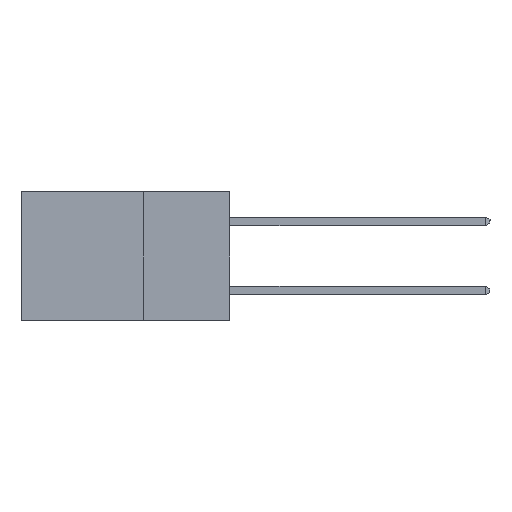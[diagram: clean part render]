
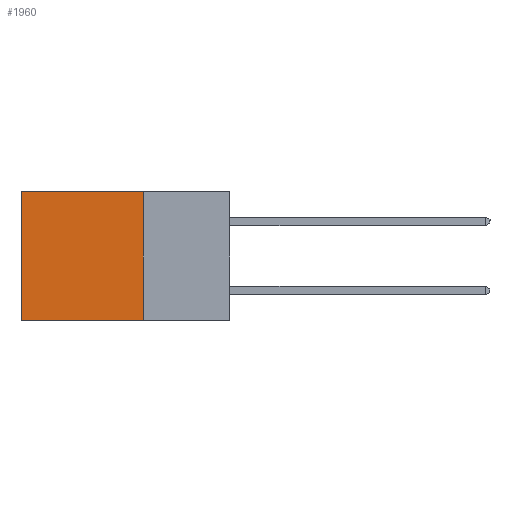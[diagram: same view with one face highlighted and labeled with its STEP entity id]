
A CAD part, left-side view. The second image highlights one B-rep face of the part: STEP entity #1960.
In plain terms, the highlighted planar face has unit normal (-1, 0, 0).
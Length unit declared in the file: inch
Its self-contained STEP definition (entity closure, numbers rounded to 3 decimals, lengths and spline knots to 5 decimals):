
#203 = EDGE_CURVE ( 'NONE', #4216, #11669, #5562, .T. ) ;
#353 = DIRECTION ( 'NONE',  ( 0., 0., -1. ) ) ;
#678 = EDGE_CURVE ( 'NONE', #3922, #4216, #9268, .T. ) ;
#1000 = EDGE_CURVE ( 'NONE', #10885, #11669, #6134, .T. ) ;
#1345 = VECTOR ( 'NONE', #6758, 39.37008 ) ;
#1960 = ADVANCED_FACE ( 'NONE', ( #9344 ), #10520, .F. ) ;
#2967 = CARTESIAN_POINT ( 'NONE',  ( 0.2615, 0.25, -0.37 ) ) ;
#3046 = CARTESIAN_POINT ( 'NONE',  ( 0.2615, 0.6, -0.37 ) ) ;
#3922 = VERTEX_POINT ( 'NONE', #4090 ) ;
#4090 = CARTESIAN_POINT ( 'NONE',  ( 0.2615, 0.25, 0. ) ) ;
#4141 = ORIENTED_EDGE ( 'NONE', *, *, #678, .T. ) ;
#4216 = VERTEX_POINT ( 'NONE', #12149 ) ;
#4281 = CARTESIAN_POINT ( 'NONE',  ( 0.2615, 0.25, 0. ) ) ;
#4487 = DIRECTION ( 'NONE',  ( 1., 0., 0. ) ) ;
#4678 = VECTOR ( 'NONE', #10916, 39.37008 ) ;
#5361 = CARTESIAN_POINT ( 'NONE',  ( 0.2615, 0.6, -0.37 ) ) ;
#5562 = LINE ( 'NONE', #5361, #6367 ) ;
#5993 = AXIS2_PLACEMENT_3D ( 'NONE', #11315, #4487, #6482 ) ;
#6134 = LINE ( 'NONE', #2967, #4678 ) ;
#6367 = VECTOR ( 'NONE', #353, 39.37008 ) ;
#6482 = DIRECTION ( 'NONE',  ( 0., 0., -1. ) ) ;
#6573 = VECTOR ( 'NONE', #12506, 39.37008 ) ;
#6758 = DIRECTION ( 'NONE',  ( 0., 0., -1. ) ) ;
#6778 = ORIENTED_EDGE ( 'NONE', *, *, #1000, .F. ) ;
#6894 = LINE ( 'NONE', #8849, #1345 ) ;
#7166 = EDGE_LOOP ( 'NONE', ( #10485, #6778, #12826, #4141 ) ) ;
#8849 = CARTESIAN_POINT ( 'NONE',  ( 0.2615, 0.25, -0.37 ) ) ;
#9268 = LINE ( 'NONE', #4281, #6573 ) ;
#9344 = FACE_OUTER_BOUND ( 'NONE', #7166, .T. ) ;
#10311 = EDGE_CURVE ( 'NONE', #3922, #10885, #6894, .T. ) ;
#10485 = ORIENTED_EDGE ( 'NONE', *, *, #203, .T. ) ;
#10520 = PLANE ( 'NONE',  #5993 ) ;
#10885 = VERTEX_POINT ( 'NONE', #12774 ) ;
#10916 = DIRECTION ( 'NONE',  ( 0., 1., 0. ) ) ;
#11315 = CARTESIAN_POINT ( 'NONE',  ( 0.2615, 0.25, -0.37 ) ) ;
#11669 = VERTEX_POINT ( 'NONE', #3046 ) ;
#12149 = CARTESIAN_POINT ( 'NONE',  ( 0.2615, 0.6, 0. ) ) ;
#12506 = DIRECTION ( 'NONE',  ( 0., 1., 0. ) ) ;
#12774 = CARTESIAN_POINT ( 'NONE',  ( 0.2615, 0.25, -0.37 ) ) ;
#12826 = ORIENTED_EDGE ( 'NONE', *, *, #10311, .F. ) ;
